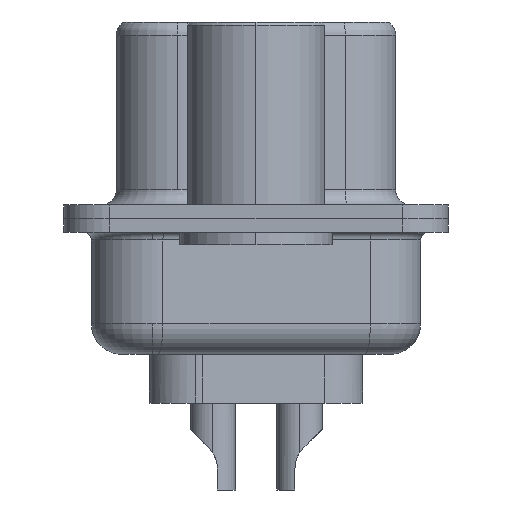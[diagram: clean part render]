
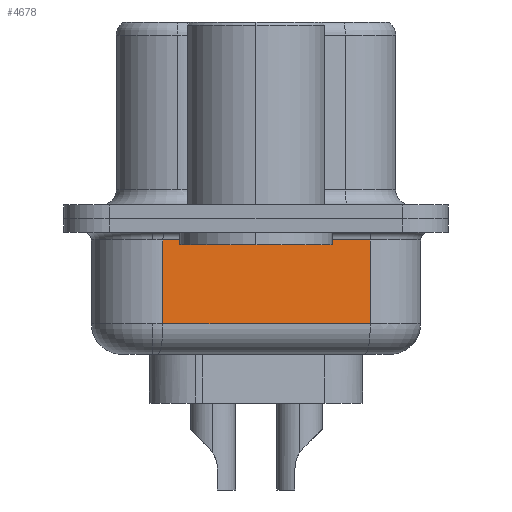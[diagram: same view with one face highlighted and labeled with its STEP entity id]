
A CAD part, left-side view. The second image highlights one B-rep face of the part: STEP entity #4678.
In plain terms, the highlighted planar face has unit normal (-0.985, -0.174, 0).
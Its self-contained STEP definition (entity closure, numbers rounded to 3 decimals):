
#107 = CARTESIAN_POINT ( 'NONE',  ( 4.089, -3.747, -3.45 ) ) ;
#398 = DIRECTION ( 'NONE',  ( 0.174, -0.985, 0. ) ) ;
#643 = DIRECTION ( 'NONE',  ( 0.985, 0.174, 0. ) ) ;
#2036 = VERTEX_POINT ( 'NONE', #15169 ) ;
#2906 = CARTESIAN_POINT ( 'NONE',  ( 2.89, 3.053, -4.45 ) ) ;
#4020 = AXIS2_PLACEMENT_3D ( 'NONE', #9724, #643, #11258 ) ;
#4354 = LINE ( 'NONE', #19461, #11923 ) ;
#4524 = EDGE_CURVE ( 'NONE', #2036, #19462, #19116, .T. ) ;
#4678 = ADVANCED_FACE ( 'NONE', ( #12171 ), #14267, .F. ) ;
#5011 = EDGE_CURVE ( 'NONE', #19462, #11403, #4354, .T. ) ;
#5042 = LINE ( 'NONE', #6063, #10943 ) ;
#6063 = CARTESIAN_POINT ( 'NONE',  ( 2.89, 3.053, -0.7 ) ) ;
#7327 = CARTESIAN_POINT ( 'NONE',  ( 4.089, -3.747, -0.7 ) ) ;
#7402 = EDGE_CURVE ( 'NONE', #11403, #7525, #5042, .T. ) ;
#7525 = VERTEX_POINT ( 'NONE', #7833 ) ;
#7833 = CARTESIAN_POINT ( 'NONE',  ( 2.89, 3.053, -0.7 ) ) ;
#7988 = CARTESIAN_POINT ( 'NONE',  ( 2.89, 3.053, -3.45 ) ) ;
#8602 = LINE ( 'NONE', #2906, #9083 ) ;
#8636 = ORIENTED_EDGE ( 'NONE', *, *, #18917, .F. ) ;
#9083 = VECTOR ( 'NONE', #11976, 1000. ) ;
#9597 = ORIENTED_EDGE ( 'NONE', *, *, #4524, .T. ) ;
#9724 = CARTESIAN_POINT ( 'NONE',  ( 2.89, 3.053, -4.45 ) ) ;
#10943 = VECTOR ( 'NONE', #18146, 1000. ) ;
#11258 = DIRECTION ( 'NONE',  ( -0.174, 0.985, 0. ) ) ;
#11403 = VERTEX_POINT ( 'NONE', #7327 ) ;
#11448 = ORIENTED_EDGE ( 'NONE', *, *, #5011, .T. ) ;
#11923 = VECTOR ( 'NONE', #19539, 1000. ) ;
#11976 = DIRECTION ( 'NONE',  ( 0., 0., 1. ) ) ;
#12171 = FACE_OUTER_BOUND ( 'NONE', #17586, .T. ) ;
#13995 = ORIENTED_EDGE ( 'NONE', *, *, #7402, .T. ) ;
#14267 = PLANE ( 'NONE',  #4020 ) ;
#15169 = CARTESIAN_POINT ( 'NONE',  ( 2.89, 3.053, -3.45 ) ) ;
#15542 = VECTOR ( 'NONE', #398, 1000. ) ;
#17586 = EDGE_LOOP ( 'NONE', ( #8636, #9597, #11448, #13995 ) ) ;
#18146 = DIRECTION ( 'NONE',  ( -0.174, 0.985, 0. ) ) ;
#18917 = EDGE_CURVE ( 'NONE', #2036, #7525, #8602, .T. ) ;
#19116 = LINE ( 'NONE', #7988, #15542 ) ;
#19461 = CARTESIAN_POINT ( 'NONE',  ( 4.089, -3.747, -4.45 ) ) ;
#19462 = VERTEX_POINT ( 'NONE', #107 ) ;
#19539 = DIRECTION ( 'NONE',  ( 0., 0., 1. ) ) ;
